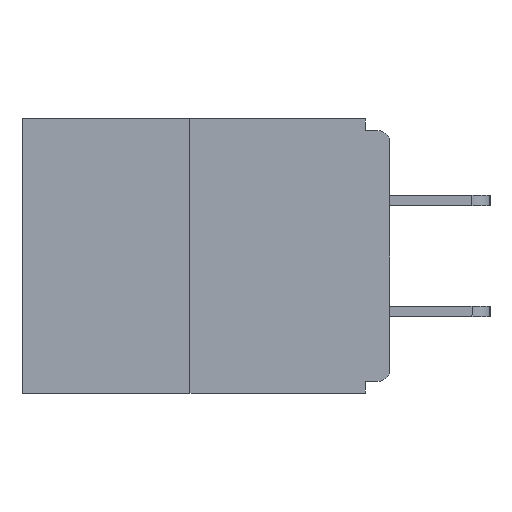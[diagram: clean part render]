
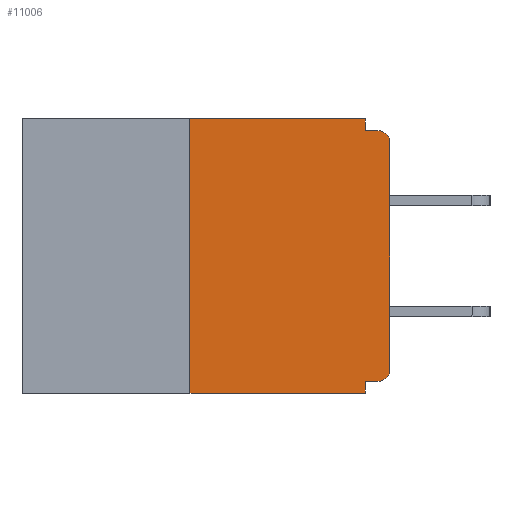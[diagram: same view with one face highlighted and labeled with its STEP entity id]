
A CAD part, left-side view. The second image highlights one B-rep face of the part: STEP entity #11006.
In plain terms, the highlighted planar face has unit normal (-1, 0, 0).
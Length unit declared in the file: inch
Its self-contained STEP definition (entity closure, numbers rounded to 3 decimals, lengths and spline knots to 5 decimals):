
#246 = CARTESIAN_POINT ( 'NONE',  ( 0., 0.031, -0.015 ) ) ;
#286 = EDGE_CURVE ( 'NONE', #9533, #1895, #11872, .T. ) ;
#300 = ORIENTED_EDGE ( 'NONE', *, *, #11426, .F. ) ;
#451 = VERTEX_POINT ( 'NONE', #7510 ) ;
#661 = CARTESIAN_POINT ( 'NONE',  ( 0., 0.015, -0.03 ) ) ;
#750 = LINE ( 'NONE', #8878, #9707 ) ;
#986 = AXIS2_PLACEMENT_3D ( 'NONE', #9242, #3513, #7319 ) ;
#1064 = DIRECTION ( 'NONE',  ( 0., 0., -1. ) ) ;
#1112 = LINE ( 'NONE', #10615, #8298 ) ;
#1151 = VERTEX_POINT ( 'NONE', #4192 ) ;
#1186 = EDGE_CURVE ( 'NONE', #8708, #1895, #9227, .T. ) ;
#1430 = CARTESIAN_POINT ( 'NONE',  ( 0., 0.25, 0. ) ) ;
#1577 = CARTESIAN_POINT ( 'NONE',  ( 0., 0., -0.03 ) ) ;
#1747 = EDGE_CURVE ( 'NONE', #11492, #1151, #2178, .T. ) ;
#1895 = VERTEX_POINT ( 'NONE', #11093 ) ;
#2178 = CIRCLE ( 'NONE', #986, 0.015 ) ;
#2251 = DIRECTION ( 'NONE',  ( 0., -1., 0. ) ) ;
#2578 = ORIENTED_EDGE ( 'NONE', *, *, #9433, .F. ) ;
#2631 = DIRECTION ( 'NONE',  ( -1., 0., 0. ) ) ;
#3019 = CARTESIAN_POINT ( 'NONE',  ( 0., 0.25, 0. ) ) ;
#3161 = EDGE_CURVE ( 'NONE', #1151, #9533, #1112, .T. ) ;
#3401 = ORIENTED_EDGE ( 'NONE', *, *, #5794, .F. ) ;
#3462 = EDGE_CURVE ( 'NONE', #11808, #8708, #8288, .T. ) ;
#3513 = DIRECTION ( 'NONE',  ( -1., 0., 0. ) ) ;
#3600 = VECTOR ( 'NONE', #11802, 39.37008 ) ;
#3659 = VERTEX_POINT ( 'NONE', #1430 ) ;
#3774 = ORIENTED_EDGE ( 'NONE', *, *, #286, .T. ) ;
#3868 = CARTESIAN_POINT ( 'NONE',  ( 0., 0.031, 0. ) ) ;
#3903 = DIRECTION ( 'NONE',  ( 0., 1., 0. ) ) ;
#3947 = ORIENTED_EDGE ( 'NONE', *, *, #3161, .T. ) ;
#3966 = CARTESIAN_POINT ( 'NONE',  ( 0., 0.031, -0.343 ) ) ;
#4192 = CARTESIAN_POINT ( 'NONE',  ( 0., 0., -0.313 ) ) ;
#4267 = DIRECTION ( 'NONE',  ( 0., -1., 0. ) ) ;
#4739 = ORIENTED_EDGE ( 'NONE', *, *, #1747, .T. ) ;
#5071 = VERTEX_POINT ( 'NONE', #11839 ) ;
#5335 = VERTEX_POINT ( 'NONE', #8413 ) ;
#5401 = AXIS2_PLACEMENT_3D ( 'NONE', #661, #2631, #9272 ) ;
#5521 = LINE ( 'NONE', #3019, #7160 ) ;
#5649 = FACE_OUTER_BOUND ( 'NONE', #11232, .T. ) ;
#5789 = DIRECTION ( 'NONE',  ( 0., 0., 1. ) ) ;
#5794 = EDGE_CURVE ( 'NONE', #3659, #11808, #750, .T. ) ;
#5882 = DIRECTION ( 'NONE',  ( 1., 0., 0. ) ) ;
#6125 = CARTESIAN_POINT ( 'NONE',  ( 0., 0.46, -0.343 ) ) ;
#6690 = ORIENTED_EDGE ( 'NONE', *, *, #8396, .T. ) ;
#7158 = VECTOR ( 'NONE', #9255, 39.37008 ) ;
#7160 = VECTOR ( 'NONE', #5789, 39.37008 ) ;
#7319 = DIRECTION ( 'NONE',  ( 0., 0., -1. ) ) ;
#7510 = CARTESIAN_POINT ( 'NONE',  ( 0., 0.031, -0.343 ) ) ;
#7626 = EDGE_CURVE ( 'NONE', #5071, #451, #7780, .T. ) ;
#7646 = VECTOR ( 'NONE', #2251, 39.37008 ) ;
#7694 = CARTESIAN_POINT ( 'NONE',  ( 0., 0.46, 0. ) ) ;
#7780 = LINE ( 'NONE', #3966, #10811 ) ;
#8014 = CARTESIAN_POINT ( 'NONE',  ( 0., 0., -0.015 ) ) ;
#8288 = LINE ( 'NONE', #11195, #7158 ) ;
#8298 = VECTOR ( 'NONE', #9760, 39.37008 ) ;
#8396 = EDGE_CURVE ( 'NONE', #5335, #451, #10351, .T. ) ;
#8413 = CARTESIAN_POINT ( 'NONE',  ( 0., 0.25, -0.343 ) ) ;
#8512 = DIRECTION ( 'NONE',  ( 0., 0., -1. ) ) ;
#8615 = CARTESIAN_POINT ( 'NONE',  ( 0., 0., -0.328 ) ) ;
#8663 = VECTOR ( 'NONE', #3903, 39.37008 ) ;
#8708 = VERTEX_POINT ( 'NONE', #246 ) ;
#8878 = CARTESIAN_POINT ( 'NONE',  ( 0., 0.46, 0. ) ) ;
#8902 = AXIS2_PLACEMENT_3D ( 'NONE', #7694, #5882, #1064 ) ;
#9020 = CARTESIAN_POINT ( 'NONE',  ( 0., 0.015, -0.328 ) ) ;
#9227 = LINE ( 'NONE', #8014, #7646 ) ;
#9242 = CARTESIAN_POINT ( 'NONE',  ( 0., 0.015, -0.313 ) ) ;
#9255 = DIRECTION ( 'NONE',  ( 0., 0., -1. ) ) ;
#9272 = DIRECTION ( 'NONE',  ( 0., 0., -1. ) ) ;
#9286 = ORIENTED_EDGE ( 'NONE', *, *, #3462, .F. ) ;
#9433 = EDGE_CURVE ( 'NONE', #5335, #3659, #5521, .T. ) ;
#9533 = VERTEX_POINT ( 'NONE', #1577 ) ;
#9707 = VECTOR ( 'NONE', #4267, 39.37008 ) ;
#9760 = DIRECTION ( 'NONE',  ( 0., 0., 1. ) ) ;
#10351 = LINE ( 'NONE', #6125, #3600 ) ;
#10615 = CARTESIAN_POINT ( 'NONE',  ( 0., 0., 0. ) ) ;
#10706 = LINE ( 'NONE', #8615, #8663 ) ;
#10802 = ORIENTED_EDGE ( 'NONE', *, *, #7626, .F. ) ;
#10811 = VECTOR ( 'NONE', #8512, 39.37008 ) ;
#10849 = PLANE ( 'NONE',  #8902 ) ;
#10933 = ORIENTED_EDGE ( 'NONE', *, *, #1186, .F. ) ;
#11006 = ADVANCED_FACE ( 'NONE', ( #5649 ), #10849, .F. ) ;
#11093 = CARTESIAN_POINT ( 'NONE',  ( 0., 0.015, -0.015 ) ) ;
#11195 = CARTESIAN_POINT ( 'NONE',  ( 0., 0.031, 0. ) ) ;
#11232 = EDGE_LOOP ( 'NONE', ( #3401, #2578, #6690, #10802, #300, #4739, #3947, #3774, #10933, #9286 ) ) ;
#11426 = EDGE_CURVE ( 'NONE', #11492, #5071, #10706, .T. ) ;
#11492 = VERTEX_POINT ( 'NONE', #9020 ) ;
#11802 = DIRECTION ( 'NONE',  ( 0., -1., 0. ) ) ;
#11808 = VERTEX_POINT ( 'NONE', #3868 ) ;
#11839 = CARTESIAN_POINT ( 'NONE',  ( 0., 0.031, -0.328 ) ) ;
#11872 = CIRCLE ( 'NONE', #5401, 0.015 ) ;
